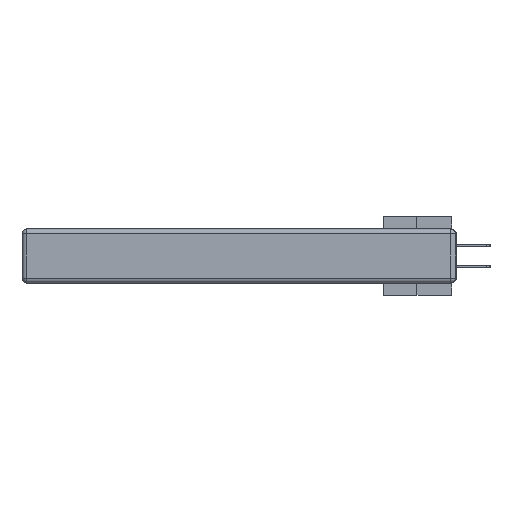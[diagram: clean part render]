
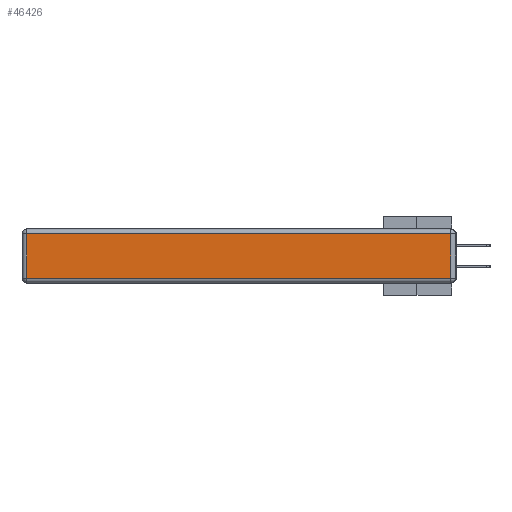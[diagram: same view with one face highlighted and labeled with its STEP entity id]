
A CAD part, left-side view. The second image highlights one B-rep face of the part: STEP entity #46426.
In plain terms, the highlighted planar face has unit normal (-1, 0, 0).
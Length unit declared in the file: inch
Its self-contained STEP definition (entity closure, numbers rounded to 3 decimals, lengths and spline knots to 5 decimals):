
#448 = DIRECTION ( 'NONE',  ( 0., 0., 1. ) ) ;
#524 = DIRECTION ( 'NONE',  ( 0., 0., -1. ) ) ;
#2861 = EDGE_CURVE ( 'NONE', #15836, #33422, #28449, .T. ) ;
#2924 = DIRECTION ( 'NONE',  ( 0., -1., 0. ) ) ;
#3125 = VECTOR ( 'NONE', #448, 39.37008 ) ;
#6365 = ORIENTED_EDGE ( 'NONE', *, *, #2861, .T. ) ;
#7683 = ORIENTED_EDGE ( 'NONE', *, *, #19357, .T. ) ;
#7935 = CARTESIAN_POINT ( 'NONE',  ( 0., 2.72, -0.313 ) ) ;
#10268 = LINE ( 'NONE', #25641, #27322 ) ;
#13390 = VECTOR ( 'NONE', #27399, 39.37008 ) ;
#14927 = AXIS2_PLACEMENT_3D ( 'NONE', #24817, #32139, #28451 ) ;
#15836 = VERTEX_POINT ( 'NONE', #7935 ) ;
#16581 = CARTESIAN_POINT ( 'NONE',  ( 0., 0.03, -0.313 ) ) ;
#19357 = EDGE_CURVE ( 'NONE', #38362, #29313, #22570, .T. ) ;
#20742 = CARTESIAN_POINT ( 'NONE',  ( 0., 0., -0.313 ) ) ;
#21833 = EDGE_LOOP ( 'NONE', ( #6365, #40563, #7683, #47163 ) ) ;
#22570 = LINE ( 'NONE', #45981, #13390 ) ;
#23606 = LINE ( 'NONE', #33182, #3125 ) ;
#24817 = CARTESIAN_POINT ( 'NONE',  ( 0., 0., -0.343 ) ) ;
#25641 = CARTESIAN_POINT ( 'NONE',  ( 0., 2.72, -0.343 ) ) ;
#27322 = VECTOR ( 'NONE', #524, 39.37008 ) ;
#27399 = DIRECTION ( 'NONE',  ( 0., 1., 0. ) ) ;
#28449 = LINE ( 'NONE', #20742, #39282 ) ;
#28451 = DIRECTION ( 'NONE',  ( 0., 0., 1. ) ) ;
#28569 = CARTESIAN_POINT ( 'NONE',  ( 0., 0.03, -0.03 ) ) ;
#29313 = VERTEX_POINT ( 'NONE', #34311 ) ;
#30455 = EDGE_CURVE ( 'NONE', #33422, #38362, #23606, .T. ) ;
#32139 = DIRECTION ( 'NONE',  ( -1., 0., 0. ) ) ;
#33182 = CARTESIAN_POINT ( 'NONE',  ( 0., 0.03, -0.343 ) ) ;
#33422 = VERTEX_POINT ( 'NONE', #16581 ) ;
#34311 = CARTESIAN_POINT ( 'NONE',  ( 0., 2.72, -0.03 ) ) ;
#38109 = EDGE_CURVE ( 'NONE', #29313, #15836, #10268, .T. ) ;
#38362 = VERTEX_POINT ( 'NONE', #28569 ) ;
#38395 = FACE_OUTER_BOUND ( 'NONE', #21833, .T. ) ;
#39282 = VECTOR ( 'NONE', #2924, 39.37008 ) ;
#40563 = ORIENTED_EDGE ( 'NONE', *, *, #30455, .T. ) ;
#42626 = PLANE ( 'NONE',  #14927 ) ;
#45981 = CARTESIAN_POINT ( 'NONE',  ( 0., 2.75, -0.03 ) ) ;
#46426 = ADVANCED_FACE ( 'NONE', ( #38395 ), #42626, .T. ) ;
#47163 = ORIENTED_EDGE ( 'NONE', *, *, #38109, .T. ) ;
